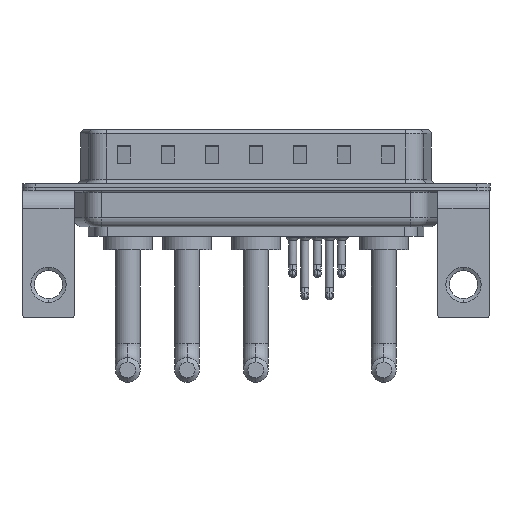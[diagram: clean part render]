
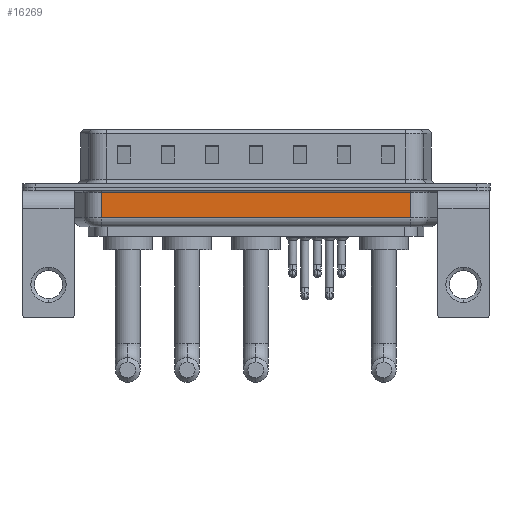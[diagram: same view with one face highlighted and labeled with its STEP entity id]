
A CAD part, front view. The second image highlights one B-rep face of the part: STEP entity #16269.
In plain terms, the highlighted planar face has unit normal (0, -1, 0).
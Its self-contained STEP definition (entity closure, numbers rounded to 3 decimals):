
#785 = LINE ( 'NONE', #7965, #1985 ) ;
#996 = CARTESIAN_POINT ( 'NONE',  ( 6.006, -5.35, -3.5 ) ) ;
#1088 = DIRECTION ( 'NONE',  ( 0., 1., 0. ) ) ;
#1885 = ORIENTED_EDGE ( 'NONE', *, *, #23114, .F. ) ;
#1985 = VECTOR ( 'NONE', #15308, 1000. ) ;
#2432 = EDGE_CURVE ( 'NONE', #9126, #21475, #5867, .T. ) ;
#3089 = PLANE ( 'NONE',  #13266 ) ;
#3653 = DIRECTION ( 'NONE',  ( 0., 0., 1. ) ) ;
#4432 = ORIENTED_EDGE ( 'NONE', *, *, #2432, .T. ) ;
#4797 = VECTOR ( 'NONE', #3653, 1000. ) ;
#5644 = LINE ( 'NONE', #19968, #21418 ) ;
#5867 = LINE ( 'NONE', #23334, #15590 ) ;
#7554 = CARTESIAN_POINT ( 'NONE',  ( 6.006, -5.35, -0.65 ) ) ;
#7965 = CARTESIAN_POINT ( 'NONE',  ( 6.006, -5.35, -3.5 ) ) ;
#8262 = DIRECTION ( 'NONE',  ( 0., 0., 1. ) ) ;
#9126 = VERTEX_POINT ( 'NONE', #20570 ) ;
#10262 = CARTESIAN_POINT ( 'NONE',  ( 6.006, -5.35, -4.5 ) ) ;
#10498 = ORIENTED_EDGE ( 'NONE', *, *, #23373, .T. ) ;
#11304 = DIRECTION ( 'NONE',  ( 0., 0., 1. ) ) ;
#13266 = AXIS2_PLACEMENT_3D ( 'NONE', #10262, #1088, #8262 ) ;
#14313 = DIRECTION ( 'NONE',  ( -1., 0., 0. ) ) ;
#15308 = DIRECTION ( 'NONE',  ( 1., 0., 0. ) ) ;
#15590 = VECTOR ( 'NONE', #14313, 1000. ) ;
#16269 = ADVANCED_FACE ( 'NONE', ( #17264 ), #3089, .F. ) ;
#16312 = CARTESIAN_POINT ( 'NONE',  ( 41.044, -5.35, -3.5 ) ) ;
#17144 = EDGE_CURVE ( 'NONE', #17574, #22743, #785, .T. ) ;
#17264 = FACE_OUTER_BOUND ( 'NONE', #20920, .T. ) ;
#17574 = VERTEX_POINT ( 'NONE', #996 ) ;
#17829 = LINE ( 'NONE', #21402, #4797 ) ;
#18710 = ORIENTED_EDGE ( 'NONE', *, *, #17144, .T. ) ;
#19968 = CARTESIAN_POINT ( 'NONE',  ( 41.044, -5.35, -4.5 ) ) ;
#20570 = CARTESIAN_POINT ( 'NONE',  ( 41.044, -5.35, -0.65 ) ) ;
#20920 = EDGE_LOOP ( 'NONE', ( #1885, #18710, #10498, #4432 ) ) ;
#21402 = CARTESIAN_POINT ( 'NONE',  ( 6.006, -5.35, -4.5 ) ) ;
#21418 = VECTOR ( 'NONE', #11304, 1000. ) ;
#21475 = VERTEX_POINT ( 'NONE', #7554 ) ;
#22743 = VERTEX_POINT ( 'NONE', #16312 ) ;
#23114 = EDGE_CURVE ( 'NONE', #17574, #21475, #17829, .T. ) ;
#23334 = CARTESIAN_POINT ( 'NONE',  ( 6.006, -5.35, -0.65 ) ) ;
#23373 = EDGE_CURVE ( 'NONE', #22743, #9126, #5644, .T. ) ;
